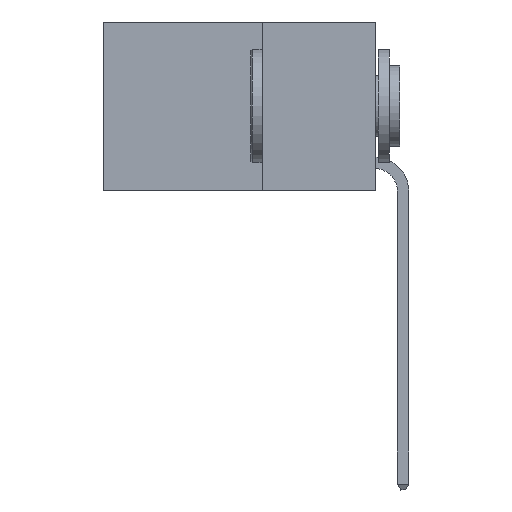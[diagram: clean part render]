
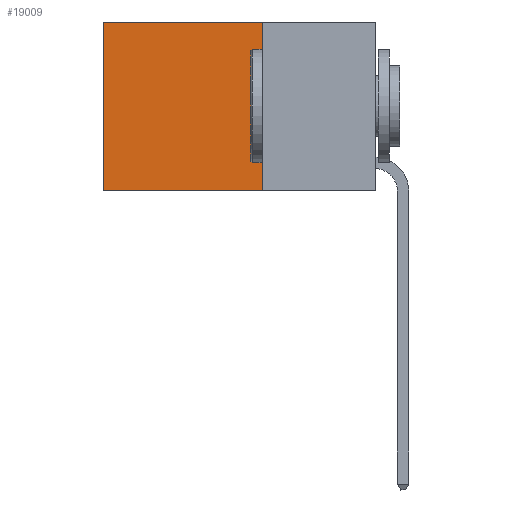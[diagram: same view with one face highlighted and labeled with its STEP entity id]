
A CAD part, left-side view. The second image highlights one B-rep face of the part: STEP entity #19009.
In plain terms, the highlighted planar face has unit normal (-1, 0, 0).
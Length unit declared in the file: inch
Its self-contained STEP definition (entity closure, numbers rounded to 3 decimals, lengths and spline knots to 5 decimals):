
#106 = DIRECTION ( 'NONE',  ( 0., 0., -1. ) ) ;
#242 = VERTEX_POINT ( 'NONE', #28954 ) ;
#2617 = FACE_OUTER_BOUND ( 'NONE', #11765, .T. ) ;
#2886 = EDGE_CURVE ( 'NONE', #242, #17363, #5929, .T. ) ;
#4739 = CARTESIAN_POINT ( 'NONE',  ( 0.2625, 0.25, 0. ) ) ;
#5929 = LINE ( 'NONE', #22467, #11403 ) ;
#6973 = EDGE_CURVE ( 'NONE', #26985, #242, #21434, .T. ) ;
#7197 = LINE ( 'NONE', #7660, #24543 ) ;
#7526 = CARTESIAN_POINT ( 'NONE',  ( 0.2625, 0.25, 0. ) ) ;
#7660 = CARTESIAN_POINT ( 'NONE',  ( 0.2625, 0.6, 0. ) ) ;
#9304 = DIRECTION ( 'NONE',  ( 0., 0., -1. ) ) ;
#9364 = DIRECTION ( 'NONE',  ( 0., 1., 0. ) ) ;
#9899 = DIRECTION ( 'NONE',  ( 1., 0., 0. ) ) ;
#10647 = ORIENTED_EDGE ( 'NONE', *, *, #6973, .F. ) ;
#10735 = ORIENTED_EDGE ( 'NONE', *, *, #2886, .F. ) ;
#10802 = EDGE_CURVE ( 'NONE', #22244, #17363, #7197, .T. ) ;
#11403 = VECTOR ( 'NONE', #17738, 39.37008 ) ;
#11765 = EDGE_LOOP ( 'NONE', ( #23821, #10735, #10647, #29268 ) ) ;
#12058 = DIRECTION ( 'NONE',  ( 0., 0., -1. ) ) ;
#14796 = CARTESIAN_POINT ( 'NONE',  ( 0.2625, 0.6, -0.37 ) ) ;
#16257 = EDGE_CURVE ( 'NONE', #26985, #22244, #23687, .T. ) ;
#17363 = VERTEX_POINT ( 'NONE', #14796 ) ;
#17738 = DIRECTION ( 'NONE',  ( 0., 1., 0. ) ) ;
#19009 = ADVANCED_FACE ( 'NONE', ( #2617 ), #21709, .F. ) ;
#19724 = CARTESIAN_POINT ( 'NONE',  ( 0.2625, 0.6, 0. ) ) ;
#21200 = CARTESIAN_POINT ( 'NONE',  ( 0.2625, 0.25, 0. ) ) ;
#21434 = LINE ( 'NONE', #30541, #25862 ) ;
#21709 = PLANE ( 'NONE',  #24093 ) ;
#22244 = VERTEX_POINT ( 'NONE', #19724 ) ;
#22467 = CARTESIAN_POINT ( 'NONE',  ( 0.2625, 0.25, -0.37 ) ) ;
#22755 = VECTOR ( 'NONE', #9364, 39.37008 ) ;
#23687 = LINE ( 'NONE', #21200, #22755 ) ;
#23821 = ORIENTED_EDGE ( 'NONE', *, *, #10802, .T. ) ;
#24093 = AXIS2_PLACEMENT_3D ( 'NONE', #7526, #9899, #106 ) ;
#24543 = VECTOR ( 'NONE', #12058, 39.37008 ) ;
#25862 = VECTOR ( 'NONE', #9304, 39.37008 ) ;
#26985 = VERTEX_POINT ( 'NONE', #4739 ) ;
#28954 = CARTESIAN_POINT ( 'NONE',  ( 0.2625, 0.25, -0.37 ) ) ;
#29268 = ORIENTED_EDGE ( 'NONE', *, *, #16257, .T. ) ;
#30541 = CARTESIAN_POINT ( 'NONE',  ( 0.2625, 0.25, 0. ) ) ;
